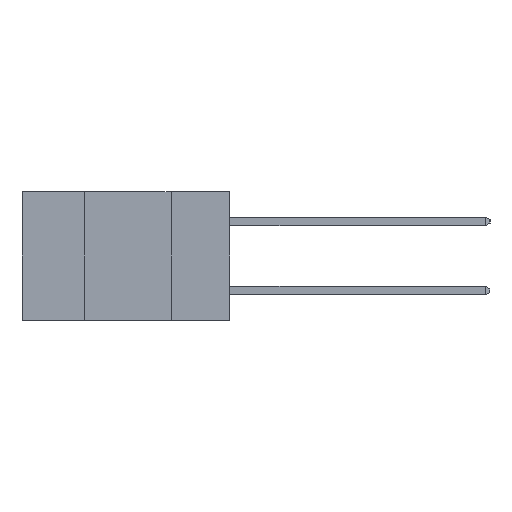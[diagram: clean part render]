
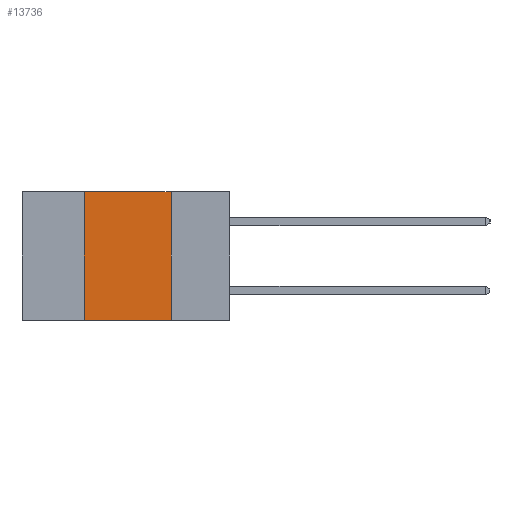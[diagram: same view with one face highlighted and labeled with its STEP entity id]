
A CAD part, left-side view. The second image highlights one B-rep face of the part: STEP entity #13736.
In plain terms, the highlighted planar face has unit normal (-1, 0, 0).
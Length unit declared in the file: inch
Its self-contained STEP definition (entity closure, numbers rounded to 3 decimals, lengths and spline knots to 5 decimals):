
#281 = CARTESIAN_POINT ( 'NONE',  ( 0., 0.6, 0. ) ) ;
#385 = LINE ( 'NONE', #5196, #4042 ) ;
#1180 = EDGE_CURVE ( 'NONE', #17310, #17566, #8782, .T. ) ;
#1927 = VERTEX_POINT ( 'NONE', #13094 ) ;
#2172 = EDGE_CURVE ( 'NONE', #1927, #13063, #10879, .T. ) ;
#2826 = CARTESIAN_POINT ( 'NONE',  ( 0., 0.42, 0. ) ) ;
#2976 = LINE ( 'NONE', #11701, #6666 ) ;
#3053 = CARTESIAN_POINT ( 'NONE',  ( 0., 0.17, 0. ) ) ;
#3504 = DIRECTION ( 'NONE',  ( 0., -1., 0. ) ) ;
#4042 = VECTOR ( 'NONE', #11987, 39.37008 ) ;
#5196 = CARTESIAN_POINT ( 'NONE',  ( 0., 0.6, 0. ) ) ;
#6150 = ORIENTED_EDGE ( 'NONE', *, *, #1180, .F. ) ;
#6416 = ORIENTED_EDGE ( 'NONE', *, *, #11943, .F. ) ;
#6620 = FACE_OUTER_BOUND ( 'NONE', #8457, .T. ) ;
#6666 = VECTOR ( 'NONE', #3504, 39.37008 ) ;
#6848 = ORIENTED_EDGE ( 'NONE', *, *, #2172, .F. ) ;
#7668 = ORIENTED_EDGE ( 'NONE', *, *, #11807, .T. ) ;
#8457 = EDGE_LOOP ( 'NONE', ( #6150, #6416, #6848, #7668 ) ) ;
#8599 = DIRECTION ( 'NONE',  ( 0., 0., -1. ) ) ;
#8782 = LINE ( 'NONE', #3053, #11937 ) ;
#9184 = CARTESIAN_POINT ( 'NONE',  ( 0., 0.17, -0.37 ) ) ;
#10879 = LINE ( 'NONE', #15009, #14420 ) ;
#11701 = CARTESIAN_POINT ( 'NONE',  ( 0., 0.6, -0.37 ) ) ;
#11807 = EDGE_CURVE ( 'NONE', #1927, #17566, #2976, .T. ) ;
#11937 = VECTOR ( 'NONE', #11978, 39.37008 ) ;
#11943 = EDGE_CURVE ( 'NONE', #13063, #17310, #385, .T. ) ;
#11978 = DIRECTION ( 'NONE',  ( 0., 0., -1. ) ) ;
#11987 = DIRECTION ( 'NONE',  ( 0., -1., 0. ) ) ;
#12778 = CARTESIAN_POINT ( 'NONE',  ( 0., 0.17, 0. ) ) ;
#13063 = VERTEX_POINT ( 'NONE', #2826 ) ;
#13094 = CARTESIAN_POINT ( 'NONE',  ( 0., 0.42, -0.37 ) ) ;
#13736 = ADVANCED_FACE ( 'NONE', ( #6620 ), #15282, .F. ) ;
#14050 = AXIS2_PLACEMENT_3D ( 'NONE', #281, #16616, #8599 ) ;
#14420 = VECTOR ( 'NONE', #16053, 39.37008 ) ;
#15009 = CARTESIAN_POINT ( 'NONE',  ( 0., 0.42, 0. ) ) ;
#15282 = PLANE ( 'NONE',  #14050 ) ;
#16053 = DIRECTION ( 'NONE',  ( 0., 0., 1. ) ) ;
#16616 = DIRECTION ( 'NONE',  ( 1., 0., 0. ) ) ;
#17310 = VERTEX_POINT ( 'NONE', #12778 ) ;
#17566 = VERTEX_POINT ( 'NONE', #9184 ) ;
